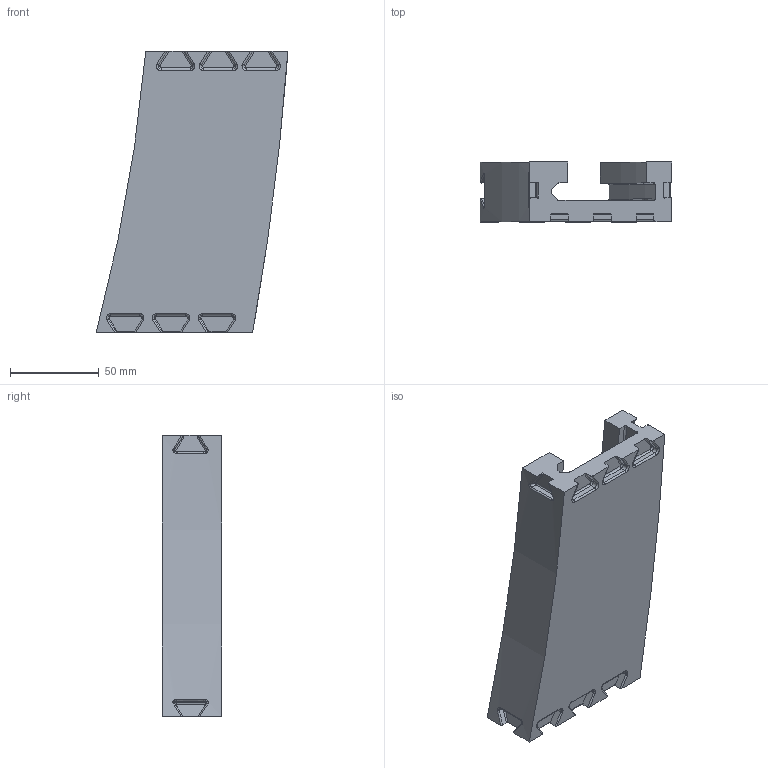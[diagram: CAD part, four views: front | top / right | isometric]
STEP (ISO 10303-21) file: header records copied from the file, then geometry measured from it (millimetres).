
FILE_DESCRIPTION(/* description */ (''),/* implementation_level */ '2;1');
FILE_NAME(/* name */ 'freeman1337-ar15-speedloader-middle-v4.step',/* time_stamp */ '2021-09-02T08:04:28-07:00',/* author */ (''),/* organization */ (''),/* preprocessor_version */ 'ST-DEVELOPER v18.1',/* originating_system */ 'Autodesk Translation Framework v10.10.0.1391',/* authorisation */ '');
FILE_SCHEMA (('AUTOMOTIVE_DESIGN { 1 0 10303 214 3 1 1 }'));
Length unit declared in the file: millimetre
Products named in the file (1): loader-middle
Bounding box: 108.23 x 33.62 x 158.74 mm (x, y, z)
Volume: 262823.1 mm3; surface area: 52578.3 mm2
Topology: 1 solids, 1 shells, 209 faces, 533 edges, 322 vertices
Faces by surface type: cylinder 81, plane 54, bspline 53, torus 21
Entity records: 7577 total; most frequent: CARTESIAN_POINT 2668, ORIENTED_EDGE 1058, DIRECTION 1011, EDGE_CURVE 529, AXIS2_PLACEMENT_3D 396, VERTEX_POINT 322, LINE 219, VECTOR 219
